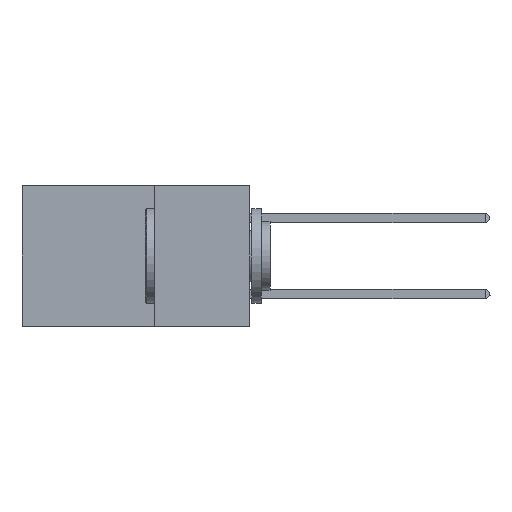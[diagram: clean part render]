
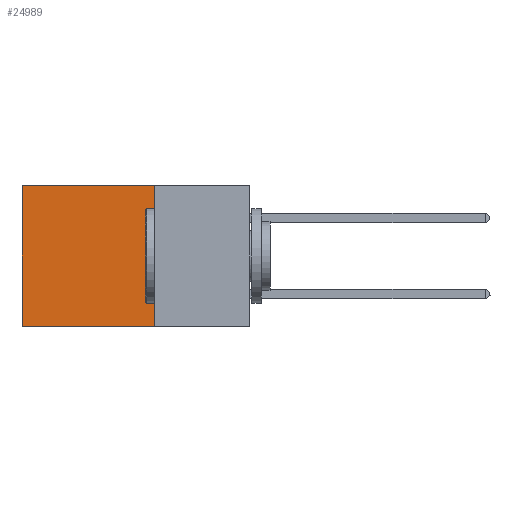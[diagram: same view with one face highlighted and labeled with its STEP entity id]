
A CAD part, left-side view. The second image highlights one B-rep face of the part: STEP entity #24989.
In plain terms, the highlighted planar face has unit normal (-1, 0, 0).
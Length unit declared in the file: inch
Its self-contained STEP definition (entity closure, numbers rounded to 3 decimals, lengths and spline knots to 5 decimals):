
#895 = ORIENTED_EDGE ( 'NONE', *, *, #24604, .T. ) ;
#950 = LINE ( 'NONE', #2416, #26419 ) ;
#1386 = DIRECTION ( 'NONE',  ( 0., 1., 0. ) ) ;
#2385 = CARTESIAN_POINT ( 'NONE',  ( 0.2875, 0.25, 0. ) ) ;
#2416 = CARTESIAN_POINT ( 'NONE',  ( 0.2875, 0.25, 0. ) ) ;
#2759 = VERTEX_POINT ( 'NONE', #2809 ) ;
#2809 = CARTESIAN_POINT ( 'NONE',  ( 0.2875, 0.6, -0.37 ) ) ;
#3298 = CARTESIAN_POINT ( 'NONE',  ( 0.2875, 0.25, 0. ) ) ;
#3394 = PLANE ( 'NONE',  #6914 ) ;
#5399 = DIRECTION ( 'NONE',  ( 1., 0., 0. ) ) ;
#6279 = LINE ( 'NONE', #22210, #25207 ) ;
#6769 = DIRECTION ( 'NONE',  ( 0., 0., -1. ) ) ;
#6914 = AXIS2_PLACEMENT_3D ( 'NONE', #3298, #5399, #9886 ) ;
#7566 = DIRECTION ( 'NONE',  ( 0., 0., -1. ) ) ;
#8306 = DIRECTION ( 'NONE',  ( 0., 1., 0. ) ) ;
#8350 = VERTEX_POINT ( 'NONE', #16129 ) ;
#8808 = LINE ( 'NONE', #14837, #11897 ) ;
#9622 = VECTOR ( 'NONE', #1386, 39.37008 ) ;
#9886 = DIRECTION ( 'NONE',  ( 0., 0., -1. ) ) ;
#11897 = VECTOR ( 'NONE', #8306, 39.37008 ) ;
#12247 = CARTESIAN_POINT ( 'NONE',  ( 0.2875, 0.25, -0.37 ) ) ;
#13158 = ORIENTED_EDGE ( 'NONE', *, *, #27894, .T. ) ;
#13865 = ORIENTED_EDGE ( 'NONE', *, *, #14093, .F. ) ;
#14093 = EDGE_CURVE ( 'NONE', #8350, #2759, #15500, .T. ) ;
#14837 = CARTESIAN_POINT ( 'NONE',  ( 0.2875, 0.25, 0. ) ) ;
#15174 = EDGE_CURVE ( 'NONE', #17726, #8350, #950, .T. ) ;
#15500 = LINE ( 'NONE', #12247, #9622 ) ;
#16129 = CARTESIAN_POINT ( 'NONE',  ( 0.2875, 0.25, -0.37 ) ) ;
#17726 = VERTEX_POINT ( 'NONE', #2385 ) ;
#21058 = VERTEX_POINT ( 'NONE', #28152 ) ;
#22210 = CARTESIAN_POINT ( 'NONE',  ( 0.2875, 0.6, 0. ) ) ;
#23399 = EDGE_LOOP ( 'NONE', ( #895, #13865, #26750, #13158 ) ) ;
#24604 = EDGE_CURVE ( 'NONE', #21058, #2759, #6279, .T. ) ;
#24989 = ADVANCED_FACE ( 'NONE', ( #27248 ), #3394, .F. ) ;
#25207 = VECTOR ( 'NONE', #6769, 39.37008 ) ;
#26419 = VECTOR ( 'NONE', #7566, 39.37008 ) ;
#26750 = ORIENTED_EDGE ( 'NONE', *, *, #15174, .F. ) ;
#27248 = FACE_OUTER_BOUND ( 'NONE', #23399, .T. ) ;
#27894 = EDGE_CURVE ( 'NONE', #17726, #21058, #8808, .T. ) ;
#28152 = CARTESIAN_POINT ( 'NONE',  ( 0.2875, 0.6, 0. ) ) ;
